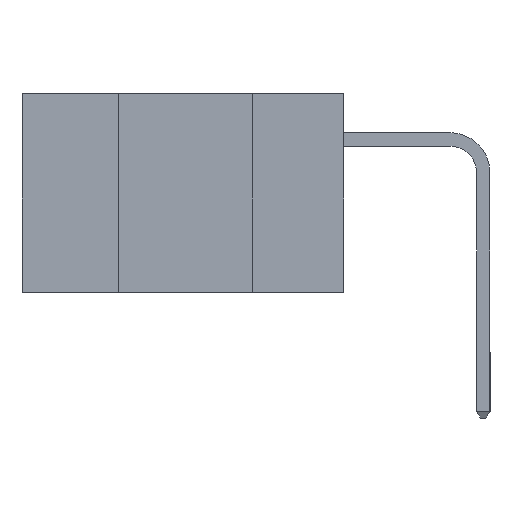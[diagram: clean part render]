
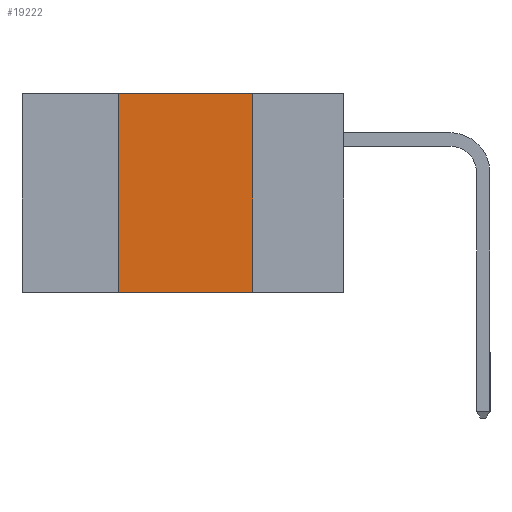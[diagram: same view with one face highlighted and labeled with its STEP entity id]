
A CAD part, left-side view. The second image highlights one B-rep face of the part: STEP entity #19222.
In plain terms, the highlighted planar face has unit normal (-1, 0, 0).
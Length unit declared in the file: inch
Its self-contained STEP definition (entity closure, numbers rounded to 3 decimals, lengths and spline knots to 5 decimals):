
#683 = CARTESIAN_POINT ( 'NONE',  ( 0., 0.6, -0.37 ) ) ;
#1840 = CARTESIAN_POINT ( 'NONE',  ( 0., 0.17, 0. ) ) ;
#2090 = EDGE_CURVE ( 'NONE', #23069, #9126, #3309, .T. ) ;
#2252 = EDGE_LOOP ( 'NONE', ( #22651, #7018, #6898, #20702 ) ) ;
#2971 = VECTOR ( 'NONE', #7088, 39.37008 ) ;
#3235 = CARTESIAN_POINT ( 'NONE',  ( 0., 0.17, -0.37 ) ) ;
#3242 = DIRECTION ( 'NONE',  ( 1., 0., 0. ) ) ;
#3309 = LINE ( 'NONE', #1840, #16030 ) ;
#3441 = EDGE_CURVE ( 'NONE', #3655, #23834, #11747, .T. ) ;
#3655 = VERTEX_POINT ( 'NONE', #11735 ) ;
#4368 = EDGE_CURVE ( 'NONE', #23834, #23069, #13724, .T. ) ;
#5669 = FACE_OUTER_BOUND ( 'NONE', #2252, .T. ) ;
#6898 = ORIENTED_EDGE ( 'NONE', *, *, #3441, .F. ) ;
#7018 = ORIENTED_EDGE ( 'NONE', *, *, #4368, .F. ) ;
#7061 = DIRECTION ( 'NONE',  ( 0., 0., -1. ) ) ;
#7088 = DIRECTION ( 'NONE',  ( 0., -1., 0. ) ) ;
#9126 = VERTEX_POINT ( 'NONE', #3235 ) ;
#9658 = VECTOR ( 'NONE', #11834, 39.37008 ) ;
#10835 = CARTESIAN_POINT ( 'NONE',  ( 0., 0.42, 0. ) ) ;
#11735 = CARTESIAN_POINT ( 'NONE',  ( 0., 0.42, -0.37 ) ) ;
#11747 = LINE ( 'NONE', #12992, #17510 ) ;
#11834 = DIRECTION ( 'NONE',  ( 0., -1., 0. ) ) ;
#12672 = DIRECTION ( 'NONE',  ( 0., 0., -1. ) ) ;
#12992 = CARTESIAN_POINT ( 'NONE',  ( 0., 0.42, 0. ) ) ;
#13724 = LINE ( 'NONE', #18119, #2971 ) ;
#14182 = CARTESIAN_POINT ( 'NONE',  ( 0., 0.6, 0. ) ) ;
#14828 = DIRECTION ( 'NONE',  ( 0., 0., 1. ) ) ;
#14925 = AXIS2_PLACEMENT_3D ( 'NONE', #14182, #3242, #7061 ) ;
#16030 = VECTOR ( 'NONE', #12672, 39.37008 ) ;
#17510 = VECTOR ( 'NONE', #14828, 39.37008 ) ;
#18119 = CARTESIAN_POINT ( 'NONE',  ( 0., 0.6, 0. ) ) ;
#19222 = ADVANCED_FACE ( 'NONE', ( #5669 ), #21580, .F. ) ;
#19796 = CARTESIAN_POINT ( 'NONE',  ( 0., 0.17, 0. ) ) ;
#20702 = ORIENTED_EDGE ( 'NONE', *, *, #21599, .T. ) ;
#21487 = LINE ( 'NONE', #683, #9658 ) ;
#21580 = PLANE ( 'NONE',  #14925 ) ;
#21599 = EDGE_CURVE ( 'NONE', #3655, #9126, #21487, .T. ) ;
#22651 = ORIENTED_EDGE ( 'NONE', *, *, #2090, .F. ) ;
#23069 = VERTEX_POINT ( 'NONE', #19796 ) ;
#23834 = VERTEX_POINT ( 'NONE', #10835 ) ;
